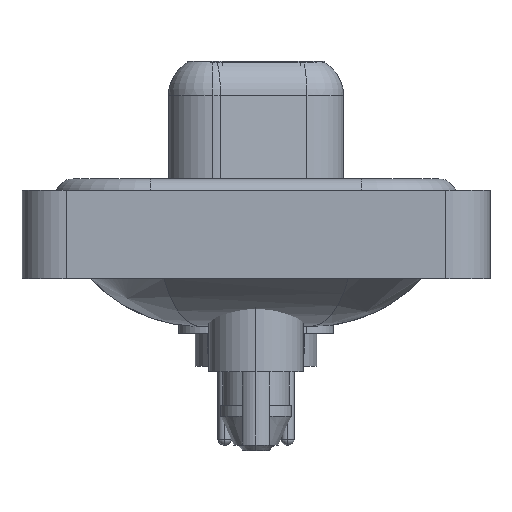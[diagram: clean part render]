
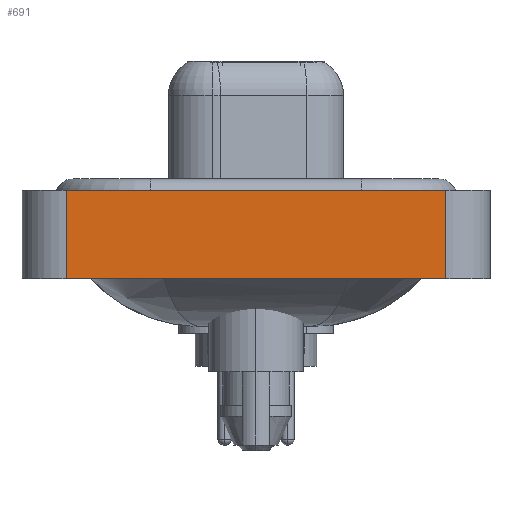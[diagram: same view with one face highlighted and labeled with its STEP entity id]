
A CAD part, left-side view. The second image highlights one B-rep face of the part: STEP entity #691.
In plain terms, the highlighted planar face has unit normal (-1, 0, 0).
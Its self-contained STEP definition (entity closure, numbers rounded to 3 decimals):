
#691 = ADVANCED_FACE ( 'NONE', ( #19500 ), #23335, .T. ) ;
#693 = DIRECTION ( 'NONE',  ( 0., -1., 0. ) ) ;
#978 = CARTESIAN_POINT ( 'NONE',  ( -7.3, 8.55, -3.6 ) ) ;
#2853 = VECTOR ( 'NONE', #7519, 1000. ) ;
#3867 = AXIS2_PLACEMENT_3D ( 'NONE', #19270, #12391, #13710 ) ;
#4424 = LINE ( 'NONE', #6464, #5269 ) ;
#5269 = VECTOR ( 'NONE', #10178, 1000. ) ;
#5752 = VERTEX_POINT ( 'NONE', #978 ) ;
#5965 = CARTESIAN_POINT ( 'NONE',  ( -7.3, -8.55, 0.4 ) ) ;
#5981 = CARTESIAN_POINT ( 'NONE',  ( -7.3, -8.55, -3.6 ) ) ;
#6464 = CARTESIAN_POINT ( 'NONE',  ( -7.3, 8.55, -3.6 ) ) ;
#7519 = DIRECTION ( 'NONE',  ( 0., -1., 0. ) ) ;
#7613 = DIRECTION ( 'NONE',  ( 0., 0., 1. ) ) ;
#7740 = CARTESIAN_POINT ( 'NONE',  ( -7.3, -8.55, -3.6 ) ) ;
#7971 = VERTEX_POINT ( 'NONE', #15009 ) ;
#8204 = ORIENTED_EDGE ( 'NONE', *, *, #10297, .T. ) ;
#9526 = LINE ( 'NONE', #7740, #13917 ) ;
#9558 = LINE ( 'NONE', #5981, #16275 ) ;
#10178 = DIRECTION ( 'NONE',  ( 0., 0., 1. ) ) ;
#10297 = EDGE_CURVE ( 'NONE', #5752, #20879, #9558, .T. ) ;
#10818 = EDGE_LOOP ( 'NONE', ( #21551, #17851, #13394, #8204 ) ) ;
#12263 = CARTESIAN_POINT ( 'NONE',  ( -7.3, -8.55, -3.6 ) ) ;
#12391 = DIRECTION ( 'NONE',  ( -1., 0., 0. ) ) ;
#13394 = ORIENTED_EDGE ( 'NONE', *, *, #20354, .F. ) ;
#13710 = DIRECTION ( 'NONE',  ( 0., 0., 1. ) ) ;
#13917 = VECTOR ( 'NONE', #7613, 1000. ) ;
#14862 = EDGE_CURVE ( 'NONE', #20879, #7971, #9526, .T. ) ;
#15009 = CARTESIAN_POINT ( 'NONE',  ( -7.3, -8.55, 0.4 ) ) ;
#16162 = VERTEX_POINT ( 'NONE', #19644 ) ;
#16275 = VECTOR ( 'NONE', #693, 1000. ) ;
#17329 = EDGE_CURVE ( 'NONE', #16162, #7971, #22410, .T. ) ;
#17851 = ORIENTED_EDGE ( 'NONE', *, *, #17329, .F. ) ;
#19270 = CARTESIAN_POINT ( 'NONE',  ( -7.3, -8.55, -3.6 ) ) ;
#19500 = FACE_OUTER_BOUND ( 'NONE', #10818, .T. ) ;
#19644 = CARTESIAN_POINT ( 'NONE',  ( -7.3, 8.55, 0.4 ) ) ;
#20354 = EDGE_CURVE ( 'NONE', #5752, #16162, #4424, .T. ) ;
#20879 = VERTEX_POINT ( 'NONE', #12263 ) ;
#21551 = ORIENTED_EDGE ( 'NONE', *, *, #14862, .T. ) ;
#22410 = LINE ( 'NONE', #5965, #2853 ) ;
#23335 = PLANE ( 'NONE',  #3867 ) ;
